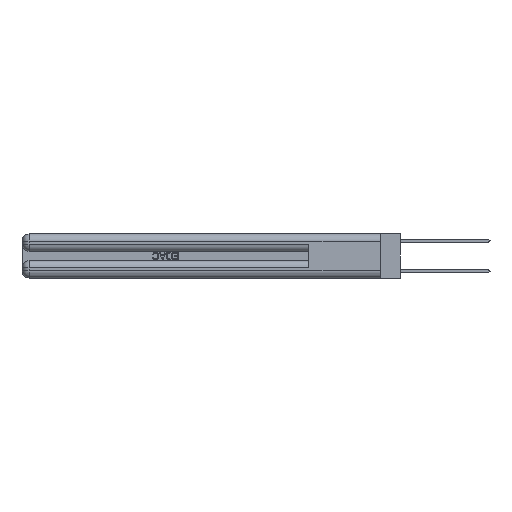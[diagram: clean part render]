
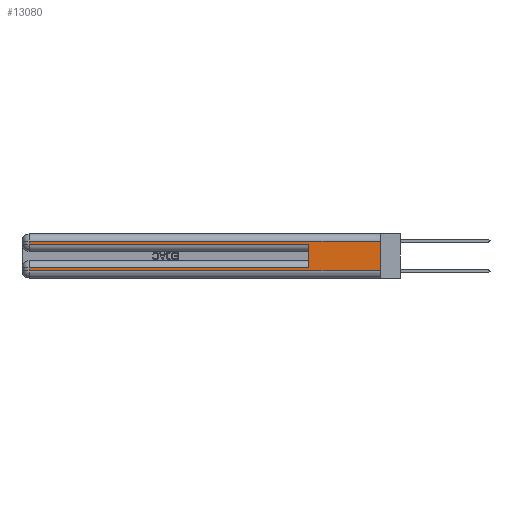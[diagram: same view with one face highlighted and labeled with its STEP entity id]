
A CAD part, left-side view. The second image highlights one B-rep face of the part: STEP entity #13080.
In plain terms, the highlighted planar face has unit normal (-1, 0, 0).
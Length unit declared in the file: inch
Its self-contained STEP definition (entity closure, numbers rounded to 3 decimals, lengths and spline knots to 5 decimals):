
#1222 = VERTEX_POINT ( 'NONE', #13579 ) ;
#1294 = LINE ( 'NONE', #10383, #28258 ) ;
#1769 = DIRECTION ( 'NONE',  ( 0., 1., 0. ) ) ;
#2913 = VECTOR ( 'NONE', #8685, 39.37008 ) ;
#3348 = LINE ( 'NONE', #18620, #16426 ) ;
#3377 = LINE ( 'NONE', #3782, #9527 ) ;
#3782 = CARTESIAN_POINT ( 'NONE',  ( 0., 0., 0.085 ) ) ;
#4350 = ORIENTED_EDGE ( 'NONE', *, *, #32889, .F. ) ;
#5372 = CARTESIAN_POINT ( 'NONE',  ( 0., 2.94, 0.285 ) ) ;
#6057 = CARTESIAN_POINT ( 'NONE',  ( 0., 0., 0.06 ) ) ;
#6265 = EDGE_CURVE ( 'NONE', #15661, #22537, #3377, .T. ) ;
#7028 = FACE_OUTER_BOUND ( 'NONE', #26429, .T. ) ;
#7342 = ORIENTED_EDGE ( 'NONE', *, *, #22323, .T. ) ;
#7912 = EDGE_CURVE ( 'NONE', #30509, #1222, #32693, .T. ) ;
#8374 = DIRECTION ( 'NONE',  ( 0., 0., 1. ) ) ;
#8677 = ORIENTED_EDGE ( 'NONE', *, *, #7912, .T. ) ;
#8685 = DIRECTION ( 'NONE',  ( 0., -1., 0. ) ) ;
#9047 = CARTESIAN_POINT ( 'NONE',  ( 0., 0., 0.285 ) ) ;
#9527 = VECTOR ( 'NONE', #11640, 39.37008 ) ;
#9637 = PLANE ( 'NONE',  #9681 ) ;
#9681 = AXIS2_PLACEMENT_3D ( 'NONE', #25231, #27863, #12245 ) ;
#9815 = ORIENTED_EDGE ( 'NONE', *, *, #6265, .T. ) ;
#10383 = CARTESIAN_POINT ( 'NONE',  ( 0., 2.94, 0.37 ) ) ;
#11640 = DIRECTION ( 'NONE',  ( 0., 1., 0. ) ) ;
#12245 = DIRECTION ( 'NONE',  ( 0., 0., -1. ) ) ;
#12574 = ORIENTED_EDGE ( 'NONE', *, *, #21183, .T. ) ;
#13080 = ADVANCED_FACE ( 'NONE', ( #7028 ), #9637, .F. ) ;
#13561 = VERTEX_POINT ( 'NONE', #32165 ) ;
#13579 = CARTESIAN_POINT ( 'NONE',  ( 0., 0.6, 0.285 ) ) ;
#13872 = VERTEX_POINT ( 'NONE', #23154 ) ;
#13877 = LINE ( 'NONE', #23923, #26108 ) ;
#13962 = EDGE_CURVE ( 'NONE', #22537, #22756, #1294, .T. ) ;
#15661 = VERTEX_POINT ( 'NONE', #28682 ) ;
#16426 = VECTOR ( 'NONE', #23837, 39.37008 ) ;
#18620 = CARTESIAN_POINT ( 'NONE',  ( 0., 2.94, 0.37 ) ) ;
#18673 = VECTOR ( 'NONE', #8374, 39.37008 ) ;
#18708 = DIRECTION ( 'NONE',  ( 0., 0., -1. ) ) ;
#20654 = ORIENTED_EDGE ( 'NONE', *, *, #30579, .T. ) ;
#21183 = EDGE_CURVE ( 'NONE', #13872, #33645, #23774, .T. ) ;
#21852 = CARTESIAN_POINT ( 'NONE',  ( 0., 2.94, 0.31 ) ) ;
#22323 = EDGE_CURVE ( 'NONE', #22756, #13561, #23736, .T. ) ;
#22537 = VERTEX_POINT ( 'NONE', #28060 ) ;
#22665 = CARTESIAN_POINT ( 'NONE',  ( 0., 0., 0.31 ) ) ;
#22756 = VERTEX_POINT ( 'NONE', #31353 ) ;
#23154 = CARTESIAN_POINT ( 'NONE',  ( 0., 0., 0.31 ) ) ;
#23736 = LINE ( 'NONE', #6057, #2913 ) ;
#23774 = LINE ( 'NONE', #22665, #29074 ) ;
#23837 = DIRECTION ( 'NONE',  ( 0., 0., -1. ) ) ;
#23923 = CARTESIAN_POINT ( 'NONE',  ( 0., 0., 0.37 ) ) ;
#24670 = DIRECTION ( 'NONE',  ( 0., -1., 0. ) ) ;
#25231 = CARTESIAN_POINT ( 'NONE',  ( 0., 0., 0.37 ) ) ;
#25583 = LINE ( 'NONE', #26496, #18673 ) ;
#26108 = VECTOR ( 'NONE', #18708, 39.37008 ) ;
#26429 = EDGE_LOOP ( 'NONE', ( #4350, #12574, #20654, #8677, #29472, #9815, #31661, #7342 ) ) ;
#26496 = CARTESIAN_POINT ( 'NONE',  ( 0., 0.6, 0.145 ) ) ;
#27835 = EDGE_CURVE ( 'NONE', #15661, #1222, #25583, .T. ) ;
#27863 = DIRECTION ( 'NONE',  ( 1., 0., 0. ) ) ;
#28060 = CARTESIAN_POINT ( 'NONE',  ( 0., 2.94, 0.085 ) ) ;
#28258 = VECTOR ( 'NONE', #31245, 39.37008 ) ;
#28682 = CARTESIAN_POINT ( 'NONE',  ( 0., 0.6, 0.085 ) ) ;
#29074 = VECTOR ( 'NONE', #1769, 39.37008 ) ;
#29472 = ORIENTED_EDGE ( 'NONE', *, *, #27835, .F. ) ;
#30509 = VERTEX_POINT ( 'NONE', #5372 ) ;
#30579 = EDGE_CURVE ( 'NONE', #33645, #30509, #3348, .T. ) ;
#31245 = DIRECTION ( 'NONE',  ( 0., 0., -1. ) ) ;
#31353 = CARTESIAN_POINT ( 'NONE',  ( 0., 2.94, 0.06 ) ) ;
#31661 = ORIENTED_EDGE ( 'NONE', *, *, #13962, .T. ) ;
#32165 = CARTESIAN_POINT ( 'NONE',  ( 0., 0., 0.06 ) ) ;
#32693 = LINE ( 'NONE', #9047, #33519 ) ;
#32889 = EDGE_CURVE ( 'NONE', #13872, #13561, #13877, .T. ) ;
#33519 = VECTOR ( 'NONE', #24670, 39.37008 ) ;
#33645 = VERTEX_POINT ( 'NONE', #21852 ) ;
